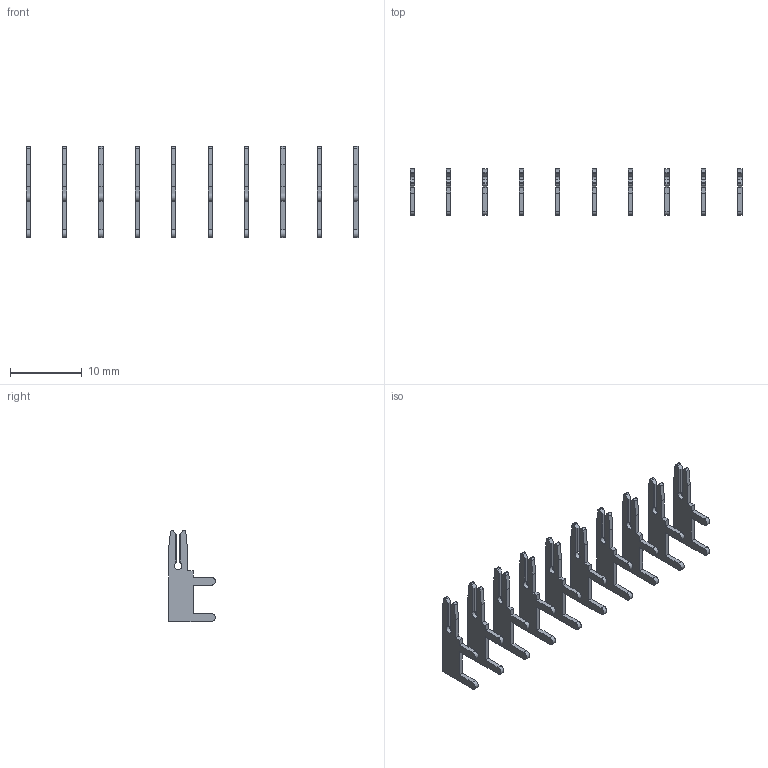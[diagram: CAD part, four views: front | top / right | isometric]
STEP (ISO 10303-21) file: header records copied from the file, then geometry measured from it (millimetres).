
FILE_DESCRIPTION (( 'STEP AP203' ), '1' );
FILE_NAME ('105-010-203-200.STEP', '2020-08-29T23:25:12', ( '' ), ( '' ), 'SwSTEP 2.0', 'SolidWorks 2020', '' );
FILE_SCHEMA (( 'CONFIG_CONTROL_DESIGN' ));
Length unit declared in the file: inch
Products named in the file (2): 100-290-001_100-290-203; 105-010-203-200
Assembly tree (10 placements, depth 2):
  105-010-203-200
    100-290-001_100-290-203  x10
Bounding box: 46.32 x 6.53 x 12.7 mm (x, y, z)
Volume: 252.5 mm3; surface area: 1157.2 mm2
Topology: 10 solids, 10 shells, 280 faces, 780 edges, 520 vertices
Faces by surface type: plane 210, cylinder 70
Entity records: 1384 total; most frequent: CARTESIAN_POINT 183, DIRECTION 170, ORIENTED_EDGE 156, EDGE_CURVE 78, VECTOR 60, LINE 60, AXIS2_PLACEMENT_3D 55, VERTEX_POINT 52
